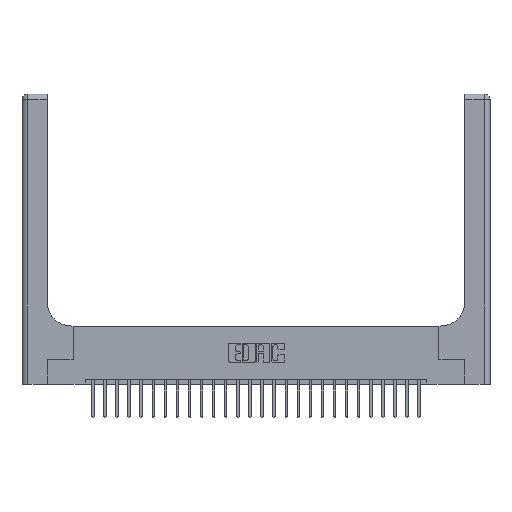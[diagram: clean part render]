
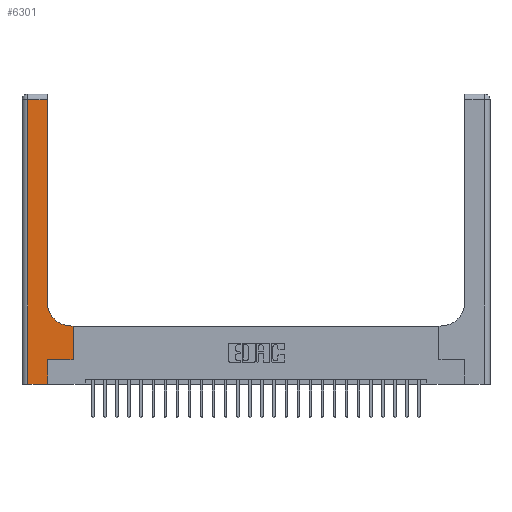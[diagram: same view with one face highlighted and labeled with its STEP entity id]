
A CAD part, top view. The second image highlights one B-rep face of the part: STEP entity #6301.
In plain terms, the highlighted planar face has unit normal (0, 0, 1).
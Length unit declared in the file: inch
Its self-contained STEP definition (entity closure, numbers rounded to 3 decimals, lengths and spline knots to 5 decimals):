
#119 = VERTEX_POINT ( 'NONE', #25221 ) ;
#308 = CARTESIAN_POINT ( 'NONE',  ( 0.528, 0.6, 0.37 ) ) ;
#365 = VECTOR ( 'NONE', #2167, 39.37008 ) ;
#417 = DIRECTION ( 'NONE',  ( 0., 1., 0. ) ) ;
#1268 = VECTOR ( 'NONE', #417, 39.37008 ) ;
#1296 = EDGE_LOOP ( 'NONE', ( #19968, #16286, #12843, #19466, #10546, #12856, #17464, #9268, #16471 ) ) ;
#1777 = AXIS2_PLACEMENT_3D ( 'NONE', #3151, #18954, #3066 ) ;
#1797 = CARTESIAN_POINT ( 'NONE',  ( 0.265, 0.25, 0.37 ) ) ;
#2145 = EDGE_CURVE ( 'NONE', #7667, #3565, #21224, .T. ) ;
#2167 = DIRECTION ( 'NONE',  ( 1., 0., 0. ) ) ;
#3066 = DIRECTION ( 'NONE',  ( -1., 0., 0. ) ) ;
#3151 = CARTESIAN_POINT ( 'NONE',  ( 0., 3., 0.37 ) ) ;
#3565 = VERTEX_POINT ( 'NONE', #16014 ) ;
#3829 = CARTESIAN_POINT ( 'NONE',  ( 0.265, 0.25, 0.37 ) ) ;
#4195 = DIRECTION ( 'NONE',  ( -1., 0., 0. ) ) ;
#4508 = LINE ( 'NONE', #15265, #17711 ) ;
#4792 = CARTESIAN_POINT ( 'NONE',  ( 0.51, 0.6, 0.37 ) ) ;
#4824 = CARTESIAN_POINT ( 'NONE',  ( 0.06, 0., 0.37 ) ) ;
#5218 = CARTESIAN_POINT ( 'NONE',  ( 0.51, 0.85, 0.37 ) ) ;
#5743 = VERTEX_POINT ( 'NONE', #20607 ) ;
#5880 = VECTOR ( 'NONE', #14399, 39.37008 ) ;
#6301 = ADVANCED_FACE ( 'NONE', ( #16733 ), #12937, .F. ) ;
#6797 = CARTESIAN_POINT ( 'NONE',  ( 0.26, 0.6, 0.37 ) ) ;
#7190 = DIRECTION ( 'NONE',  ( 1., 0., 0. ) ) ;
#7293 = DIRECTION ( 'NONE',  ( 0., 1., 0. ) ) ;
#7363 = EDGE_CURVE ( 'NONE', #16117, #5743, #7418, .T. ) ;
#7418 = LINE ( 'NONE', #1797, #5880 ) ;
#7424 = VECTOR ( 'NONE', #14104, 39.37008 ) ;
#7470 = EDGE_CURVE ( 'NONE', #11257, #7667, #22755, .T. ) ;
#7602 = EDGE_CURVE ( 'NONE', #119, #16117, #17229, .T. ) ;
#7667 = VERTEX_POINT ( 'NONE', #4792 ) ;
#7803 = VERTEX_POINT ( 'NONE', #13849 ) ;
#8280 = CARTESIAN_POINT ( 'NONE',  ( 0.06, 3., 0.37 ) ) ;
#9268 = ORIENTED_EDGE ( 'NONE', *, *, #7470, .T. ) ;
#10285 = VERTEX_POINT ( 'NONE', #12540 ) ;
#10290 = VERTEX_POINT ( 'NONE', #4824 ) ;
#10546 = ORIENTED_EDGE ( 'NONE', *, *, #7602, .T. ) ;
#10550 = VECTOR ( 'NONE', #17341, 39.37008 ) ;
#11257 = VERTEX_POINT ( 'NONE', #308 ) ;
#11552 = CARTESIAN_POINT ( 'NONE',  ( 0., 2.94, 0.37 ) ) ;
#11569 = EDGE_CURVE ( 'NONE', #3565, #10285, #13652, .T. ) ;
#12231 = AXIS2_PLACEMENT_3D ( 'NONE', #5218, #18956, #7190 ) ;
#12540 = CARTESIAN_POINT ( 'NONE',  ( 0.26, 2.94, 0.37 ) ) ;
#12843 = ORIENTED_EDGE ( 'NONE', *, *, #20751, .T. ) ;
#12856 = ORIENTED_EDGE ( 'NONE', *, *, #7363, .T. ) ;
#12937 = PLANE ( 'NONE',  #1777 ) ;
#12955 = LINE ( 'NONE', #23622, #365 ) ;
#13087 = DIRECTION ( 'NONE',  ( 0., 1., 0. ) ) ;
#13141 = EDGE_CURVE ( 'NONE', #10290, #119, #12955, .T. ) ;
#13652 = LINE ( 'NONE', #19024, #16756 ) ;
#13849 = CARTESIAN_POINT ( 'NONE',  ( 0.06, 2.94, 0.37 ) ) ;
#14104 = DIRECTION ( 'NONE',  ( 0., -1., 0. ) ) ;
#14399 = DIRECTION ( 'NONE',  ( 1., 0., 0. ) ) ;
#14780 = LINE ( 'NONE', #8280, #7424 ) ;
#15265 = CARTESIAN_POINT ( 'NONE',  ( 0.528, 0.25, 0.37 ) ) ;
#15847 = EDGE_CURVE ( 'NONE', #5743, #11257, #4508, .T. ) ;
#16014 = CARTESIAN_POINT ( 'NONE',  ( 0.26, 0.85, 0.37 ) ) ;
#16108 = CARTESIAN_POINT ( 'NONE',  ( 0.265, 0., 0.37 ) ) ;
#16117 = VERTEX_POINT ( 'NONE', #3829 ) ;
#16286 = ORIENTED_EDGE ( 'NONE', *, *, #18638, .T. ) ;
#16471 = ORIENTED_EDGE ( 'NONE', *, *, #2145, .T. ) ;
#16733 = FACE_OUTER_BOUND ( 'NONE', #1296, .T. ) ;
#16756 = VECTOR ( 'NONE', #13087, 39.37008 ) ;
#17229 = LINE ( 'NONE', #16108, #1268 ) ;
#17341 = DIRECTION ( 'NONE',  ( -1., 0., 0. ) ) ;
#17464 = ORIENTED_EDGE ( 'NONE', *, *, #15847, .T. ) ;
#17711 = VECTOR ( 'NONE', #7293, 39.37008 ) ;
#18155 = VECTOR ( 'NONE', #4195, 39.37008 ) ;
#18638 = EDGE_CURVE ( 'NONE', #10285, #7803, #20083, .T. ) ;
#18954 = DIRECTION ( 'NONE',  ( 0., 0., -1. ) ) ;
#18956 = DIRECTION ( 'NONE',  ( 0., 0., -1. ) ) ;
#19024 = CARTESIAN_POINT ( 'NONE',  ( 0.26, 3., 0.37 ) ) ;
#19466 = ORIENTED_EDGE ( 'NONE', *, *, #13141, .T. ) ;
#19968 = ORIENTED_EDGE ( 'NONE', *, *, #11569, .T. ) ;
#20083 = LINE ( 'NONE', #11552, #10550 ) ;
#20607 = CARTESIAN_POINT ( 'NONE',  ( 0.528, 0.25, 0.37 ) ) ;
#20751 = EDGE_CURVE ( 'NONE', #7803, #10290, #14780, .T. ) ;
#21224 = CIRCLE ( 'NONE', #12231, 0.25 ) ;
#22755 = LINE ( 'NONE', #6797, #18155 ) ;
#23622 = CARTESIAN_POINT ( 'NONE',  ( 0., 0., 0.37 ) ) ;
#25221 = CARTESIAN_POINT ( 'NONE',  ( 0.265, 0., 0.37 ) ) ;
